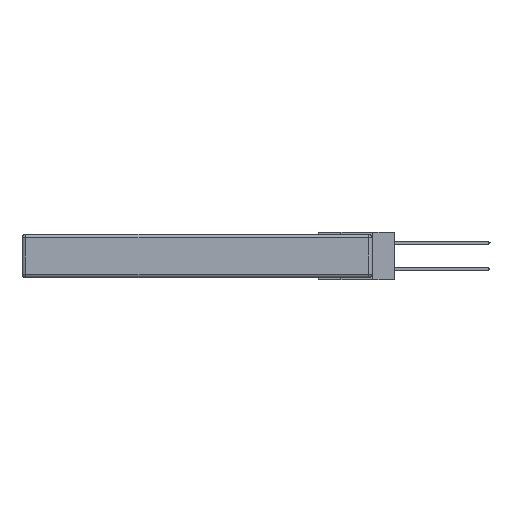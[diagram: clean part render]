
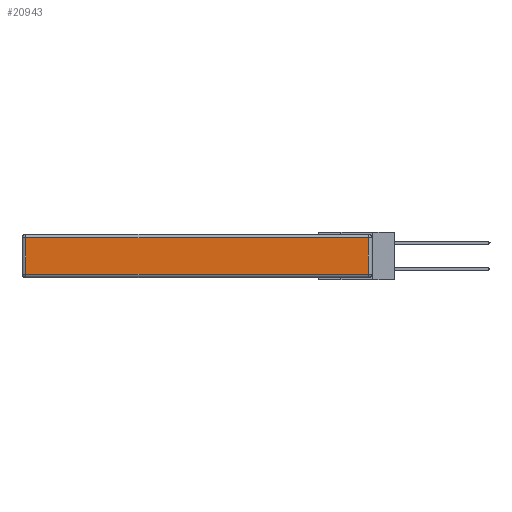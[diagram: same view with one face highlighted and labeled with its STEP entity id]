
A CAD part, left-side view. The second image highlights one B-rep face of the part: STEP entity #20943.
In plain terms, the highlighted planar face has unit normal (-1, 0, 0).
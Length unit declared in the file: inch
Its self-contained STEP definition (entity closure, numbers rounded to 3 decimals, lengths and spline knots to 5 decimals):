
#1004 = DIRECTION ( 'NONE',  ( 0., 0., 1. ) ) ;
#1136 = CARTESIAN_POINT ( 'NONE',  ( 0., 0.03, -0.343 ) ) ;
#1262 = EDGE_LOOP ( 'NONE', ( #4129, #24735, #7306, #7845 ) ) ;
#1768 = EDGE_CURVE ( 'NONE', #6310, #22258, #17639, .T. ) ;
#1957 = LINE ( 'NONE', #1975, #6748 ) ;
#1975 = CARTESIAN_POINT ( 'NONE',  ( 0., 0., -0.313 ) ) ;
#2046 = CARTESIAN_POINT ( 'NONE',  ( 0., 2.75, -0.03 ) ) ;
#2952 = CARTESIAN_POINT ( 'NONE',  ( 0., 0., -0.343 ) ) ;
#4129 = ORIENTED_EDGE ( 'NONE', *, *, #10635, .T. ) ;
#5408 = DIRECTION ( 'NONE',  ( 0., 1., 0. ) ) ;
#5500 = VECTOR ( 'NONE', #18186, 39.37008 ) ;
#6241 = DIRECTION ( 'NONE',  ( 0., -1., 0. ) ) ;
#6310 = VERTEX_POINT ( 'NONE', #18016 ) ;
#6588 = VERTEX_POINT ( 'NONE', #9895 ) ;
#6748 = VECTOR ( 'NONE', #6241, 39.37008 ) ;
#7036 = DIRECTION ( 'NONE',  ( -1., 0., 0. ) ) ;
#7306 = ORIENTED_EDGE ( 'NONE', *, *, #1768, .T. ) ;
#7845 = ORIENTED_EDGE ( 'NONE', *, *, #25533, .T. ) ;
#8310 = FACE_OUTER_BOUND ( 'NONE', #1262, .T. ) ;
#8639 = VECTOR ( 'NONE', #25490, 39.37008 ) ;
#9895 = CARTESIAN_POINT ( 'NONE',  ( 0., 0.03, -0.313 ) ) ;
#9897 = LINE ( 'NONE', #1136, #8639 ) ;
#10032 = CARTESIAN_POINT ( 'NONE',  ( 0., 2.72, -0.343 ) ) ;
#10635 = EDGE_CURVE ( 'NONE', #25348, #6588, #1957, .T. ) ;
#13452 = LINE ( 'NONE', #10032, #5500 ) ;
#13799 = VECTOR ( 'NONE', #5408, 39.37008 ) ;
#15505 = AXIS2_PLACEMENT_3D ( 'NONE', #2952, #7036, #1004 ) ;
#17377 = PLANE ( 'NONE',  #15505 ) ;
#17639 = LINE ( 'NONE', #2046, #13799 ) ;
#18016 = CARTESIAN_POINT ( 'NONE',  ( 0., 0.03, -0.03 ) ) ;
#18186 = DIRECTION ( 'NONE',  ( 0., 0., -1. ) ) ;
#19362 = CARTESIAN_POINT ( 'NONE',  ( 0., 2.72, -0.03 ) ) ;
#20464 = EDGE_CURVE ( 'NONE', #6588, #6310, #9897, .T. ) ;
#20943 = ADVANCED_FACE ( 'NONE', ( #8310 ), #17377, .T. ) ;
#21328 = CARTESIAN_POINT ( 'NONE',  ( 0., 2.72, -0.313 ) ) ;
#22258 = VERTEX_POINT ( 'NONE', #19362 ) ;
#24735 = ORIENTED_EDGE ( 'NONE', *, *, #20464, .T. ) ;
#25348 = VERTEX_POINT ( 'NONE', #21328 ) ;
#25490 = DIRECTION ( 'NONE',  ( 0., 0., 1. ) ) ;
#25533 = EDGE_CURVE ( 'NONE', #22258, #25348, #13452, .T. ) ;
